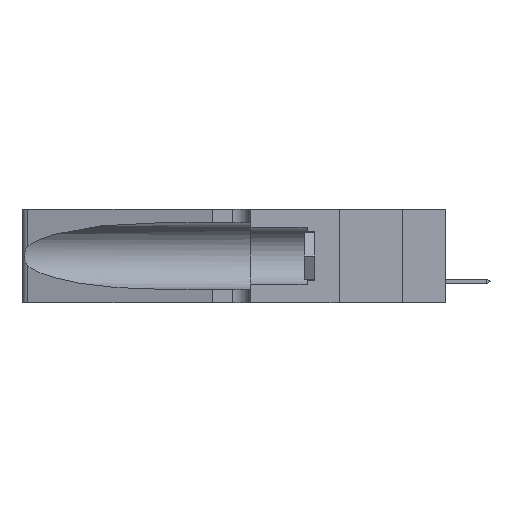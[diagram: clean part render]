
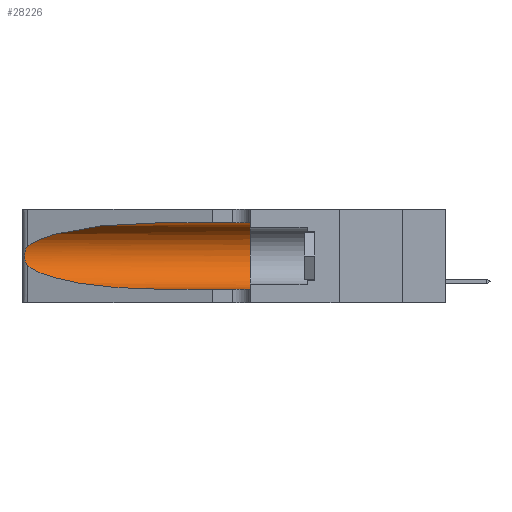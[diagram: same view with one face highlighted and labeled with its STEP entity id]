
A CAD part, left-side view. The second image highlights one B-rep face of the part: STEP entity #28226.
In plain terms, the highlighted cylindrical face has radius 3.308 mm (diameter 6.617 mm), a partial arc.
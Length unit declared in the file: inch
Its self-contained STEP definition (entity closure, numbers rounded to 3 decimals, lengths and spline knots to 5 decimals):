
#343 = DIRECTION ( 'NONE',  ( 0., -1., 0. ) ) ;
#1714 = DIRECTION ( 'NONE',  ( 0., 0., 1. ) ) ;
#2238 = EDGE_CURVE ( 'NONE', #7914, #17184, #10883, .T. ) ;
#2891 = CARTESIAN_POINT ( 'NONE',  ( 0.2373, 1.15595, 0.08982 ) ) ;
#3189 = DIRECTION ( 'NONE',  ( 0., -1., 0. ) ) ;
#3217 =( BOUNDED_CURVE ( )  B_SPLINE_CURVE ( 3, ( #30856, #2891, #35175, #10748 ),
 .UNSPECIFIED., .F., .F. ) 
 B_SPLINE_CURVE_WITH_KNOTS ( ( 4, 4 ),
 ( 3.44316, 4.71239 ),
 .UNSPECIFIED. ) 
 CURVE ( )  GEOMETRIC_REPRESENTATION_ITEM ( )  RATIONAL_B_SPLINE_CURVE ( ( 1., 0.87, 0.87, 1. ) ) 
 REPRESENTATION_ITEM ( '' )  );
#3846 = CARTESIAN_POINT ( 'NONE',  ( 0.26018, 1.23835, 0.19895 ) ) ;
#4092 = CARTESIAN_POINT ( 'NONE',  ( 0.25639, 1.23184, 0.21858 ) ) ;
#4600 = B_SPLINE_CURVE_WITH_KNOTS ( 'NONE', 3,
 ( #28198, #25682, #4092, #20302, #6323, #3846, #23157, #12289, #31394, #22803, #14789, #12171, #25438, #25808 ),
 .UNSPECIFIED., .F., .F.,
 ( 4, 2, 2, 2, 2, 2, 4 ),
 ( 0., 0.00027, 0.00053, 0.00107, 0.0016, 0.00187, 0.00214 ),
 .UNSPECIFIED. ) ;
#4666 = CARTESIAN_POINT ( 'NONE',  ( 0.25487, 1.22718, 0.14631 ) ) ;
#5283 = DIRECTION ( 'NONE',  ( 0., -1., 0. ) ) ;
#5396 = LINE ( 'NONE', #10706, #33490 ) ;
#5941 = CARTESIAN_POINT ( 'NONE',  ( 0.1305, 0.35, 0.05475 ) ) ;
#5946 = DIRECTION ( 'NONE',  ( 0., 0., -1. ) ) ;
#6129 = EDGE_CURVE ( 'NONE', #17184, #25433, #4600, .T. ) ;
#6323 = CARTESIAN_POINT ( 'NONE',  ( 0.25854, 1.2359, 0.20912 ) ) ;
#6676 = FACE_OUTER_BOUND ( 'NONE', #29702, .T. ) ;
#7914 = VERTEX_POINT ( 'NONE', #26839 ) ;
#9046 = AXIS2_PLACEMENT_3D ( 'NONE', #16652, #343, #5946 ) ;
#10411 = AXIS2_PLACEMENT_3D ( 'NONE', #34457, #29398, #1714 ) ;
#10706 = CARTESIAN_POINT ( 'NONE',  ( 0.1305, 1.61858, 0.31525 ) ) ;
#10748 = CARTESIAN_POINT ( 'NONE',  ( 0.1305, 0.72297, 0.05475 ) ) ;
#10883 =( BOUNDED_CURVE ( )  B_SPLINE_CURVE ( 3, ( #18773, #13631, #29799, #35187 ),
 .UNSPECIFIED., .F., .F. ) 
 B_SPLINE_CURVE_WITH_KNOTS ( ( 4, 4 ),
 ( 1.5708, 2.84003 ),
 .UNSPECIFIED. ) 
 CURVE ( )  GEOMETRIC_REPRESENTATION_ITEM ( )  RATIONAL_B_SPLINE_CURVE ( ( 1., 0.87, 0.87, 1. ) ) 
 REPRESENTATION_ITEM ( '' )  );
#12171 = CARTESIAN_POINT ( 'NONE',  ( 0.25639, 1.23186, 0.15144 ) ) ;
#12289 = CARTESIAN_POINT ( 'NONE',  ( 0.26075, 1.23896, 0.178 ) ) ;
#12873 = ORIENTED_EDGE ( 'NONE', *, *, #16880, .T. ) ;
#12969 = ORIENTED_EDGE ( 'NONE', *, *, #34746, .T. ) ;
#13631 = CARTESIAN_POINT ( 'NONE',  ( 0.18966, 0.96281, 0.31525 ) ) ;
#14543 = VERTEX_POINT ( 'NONE', #5941 ) ;
#14789 = CARTESIAN_POINT ( 'NONE',  ( 0.25789, 1.23486, 0.15765 ) ) ;
#16532 = ORIENTED_EDGE ( 'NONE', *, *, #2238, .T. ) ;
#16652 = CARTESIAN_POINT ( 'NONE',  ( 0.1305, 1.61858, 0.185 ) ) ;
#16880 = EDGE_CURVE ( 'NONE', #25433, #33368, #3217, .T. ) ;
#17184 = VERTEX_POINT ( 'NONE', #21122 ) ;
#18200 = ORIENTED_EDGE ( 'NONE', *, *, #6129, .T. ) ;
#18328 = VERTEX_POINT ( 'NONE', #26676 ) ;
#18773 = CARTESIAN_POINT ( 'NONE',  ( 0.1305, 0.72297, 0.31525 ) ) ;
#20302 = CARTESIAN_POINT ( 'NONE',  ( 0.25787, 1.23484, 0.2124 ) ) ;
#21122 = CARTESIAN_POINT ( 'NONE',  ( 0.25487, 1.22718, 0.22369 ) ) ;
#22666 = VECTOR ( 'NONE', #3189, 39.37008 ) ;
#22803 = CARTESIAN_POINT ( 'NONE',  ( 0.25856, 1.23593, 0.16098 ) ) ;
#23157 = CARTESIAN_POINT ( 'NONE',  ( 0.26075, 1.23896, 0.19203 ) ) ;
#24174 = CYLINDRICAL_SURFACE ( 'NONE', #9046, 0.13025 ) ;
#25161 = CIRCLE ( 'NONE', #10411, 0.13025 ) ;
#25433 = VERTEX_POINT ( 'NONE', #4666 ) ;
#25438 = CARTESIAN_POINT ( 'NONE',  ( 0.25555, 1.22993, 0.14849 ) ) ;
#25682 = CARTESIAN_POINT ( 'NONE',  ( 0.25555, 1.22994, 0.2215 ) ) ;
#25808 = CARTESIAN_POINT ( 'NONE',  ( 0.25487, 1.22718, 0.14631 ) ) ;
#26676 = CARTESIAN_POINT ( 'NONE',  ( 0.1305, 0.35, 0.31525 ) ) ;
#26839 = CARTESIAN_POINT ( 'NONE',  ( 0.1305, 0.72297, 0.31525 ) ) ;
#27076 = CARTESIAN_POINT ( 'NONE',  ( 0.1305, 0.72297, 0.05475 ) ) ;
#28198 = CARTESIAN_POINT ( 'NONE',  ( 0.25487, 1.22718, 0.22369 ) ) ;
#28226 = ADVANCED_FACE ( 'NONE', ( #6676 ), #24174, .F. ) ;
#28747 = ORIENTED_EDGE ( 'NONE', *, *, #34611, .F. ) ;
#29398 = DIRECTION ( 'NONE',  ( 0., 1., 0. ) ) ;
#29702 = EDGE_LOOP ( 'NONE', ( #16532, #18200, #12873, #12969, #32486, #28747 ) ) ;
#29799 = CARTESIAN_POINT ( 'NONE',  ( 0.2373, 1.15595, 0.28018 ) ) ;
#30856 = CARTESIAN_POINT ( 'NONE',  ( 0.25487, 1.22718, 0.14631 ) ) ;
#31394 = CARTESIAN_POINT ( 'NONE',  ( 0.26017, 1.23833, 0.17102 ) ) ;
#32486 = ORIENTED_EDGE ( 'NONE', *, *, #34551, .F. ) ;
#32546 = LINE ( 'NONE', #33102, #22666 ) ;
#33102 = CARTESIAN_POINT ( 'NONE',  ( 0.1305, 1.61858, 0.05475 ) ) ;
#33368 = VERTEX_POINT ( 'NONE', #27076 ) ;
#33490 = VECTOR ( 'NONE', #5283, 39.37008 ) ;
#34457 = CARTESIAN_POINT ( 'NONE',  ( 0.1305, 0.35, 0.185 ) ) ;
#34551 = EDGE_CURVE ( 'NONE', #18328, #14543, #25161, .T. ) ;
#34611 = EDGE_CURVE ( 'NONE', #7914, #18328, #5396, .T. ) ;
#34746 = EDGE_CURVE ( 'NONE', #33368, #14543, #32546, .T. ) ;
#35175 = CARTESIAN_POINT ( 'NONE',  ( 0.18966, 0.96281, 0.05475 ) ) ;
#35187 = CARTESIAN_POINT ( 'NONE',  ( 0.25487, 1.22718, 0.22369 ) ) ;
